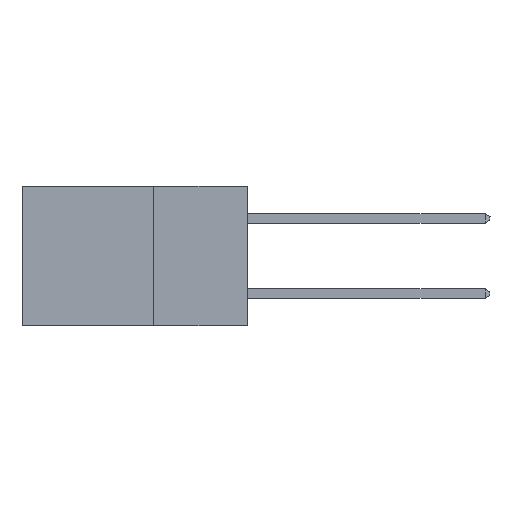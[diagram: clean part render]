
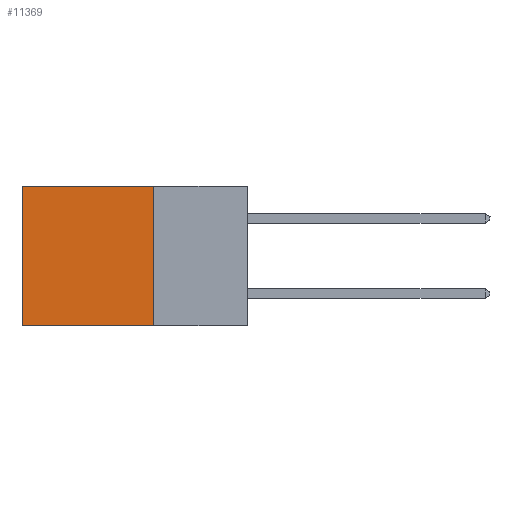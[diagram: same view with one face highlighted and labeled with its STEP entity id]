
A CAD part, left-side view. The second image highlights one B-rep face of the part: STEP entity #11369.
In plain terms, the highlighted planar face has unit normal (-1, 0, 0).
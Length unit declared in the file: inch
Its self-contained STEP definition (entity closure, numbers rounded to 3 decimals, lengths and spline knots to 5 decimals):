
#192 = DIRECTION ( 'NONE',  ( 0., 0., -1. ) ) ;
#212 = LINE ( 'NONE', #22846, #5450 ) ;
#910 = EDGE_CURVE ( 'NONE', #17585, #12472, #212, .T. ) ;
#913 = ORIENTED_EDGE ( 'NONE', *, *, #7001, .T. ) ;
#1144 = ORIENTED_EDGE ( 'NONE', *, *, #1780, .F. ) ;
#1780 = EDGE_CURVE ( 'NONE', #12472, #2490, #7830, .T. ) ;
#1997 = VECTOR ( 'NONE', #15049, 39.37008 ) ;
#2490 = VERTEX_POINT ( 'NONE', #12220 ) ;
#2828 = VERTEX_POINT ( 'NONE', #4873 ) ;
#3667 = CARTESIAN_POINT ( 'NONE',  ( 0.298, 0.6, 0. ) ) ;
#3754 = ORIENTED_EDGE ( 'NONE', *, *, #910, .F. ) ;
#4873 = CARTESIAN_POINT ( 'NONE',  ( 0.298, 0.6, 0. ) ) ;
#5029 = CARTESIAN_POINT ( 'NONE',  ( 0.298, 0.25, -0.37 ) ) ;
#5450 = VECTOR ( 'NONE', #24773, 39.37008 ) ;
#7001 = EDGE_CURVE ( 'NONE', #17585, #2828, #18368, .T. ) ;
#7830 = LINE ( 'NONE', #5029, #1997 ) ;
#8013 = PLANE ( 'NONE',  #23532 ) ;
#9423 = CARTESIAN_POINT ( 'NONE',  ( 0.298, 0.25, 0. ) ) ;
#9988 = CARTESIAN_POINT ( 'NONE',  ( 0.298, 0.25, 0. ) ) ;
#10891 = VECTOR ( 'NONE', #19261, 39.37008 ) ;
#11369 = ADVANCED_FACE ( 'NONE', ( #24390 ), #8013, .F. ) ;
#11377 = ORIENTED_EDGE ( 'NONE', *, *, #18677, .T. ) ;
#11971 = DIRECTION ( 'NONE',  ( 1., 0., 0. ) ) ;
#12220 = CARTESIAN_POINT ( 'NONE',  ( 0.298, 0.6, -0.37 ) ) ;
#12472 = VERTEX_POINT ( 'NONE', #17855 ) ;
#15049 = DIRECTION ( 'NONE',  ( 0., 1., 0. ) ) ;
#17585 = VERTEX_POINT ( 'NONE', #9423 ) ;
#17629 = DIRECTION ( 'NONE',  ( 0., 0., -1. ) ) ;
#17855 = CARTESIAN_POINT ( 'NONE',  ( 0.298, 0.25, -0.37 ) ) ;
#18368 = LINE ( 'NONE', #23260, #10891 ) ;
#18677 = EDGE_CURVE ( 'NONE', #2828, #2490, #24103, .T. ) ;
#19261 = DIRECTION ( 'NONE',  ( 0., 1., 0. ) ) ;
#22219 = VECTOR ( 'NONE', #17629, 39.37008 ) ;
#22846 = CARTESIAN_POINT ( 'NONE',  ( 0.298, 0.25, 0. ) ) ;
#23260 = CARTESIAN_POINT ( 'NONE',  ( 0.298, 0.25, 0. ) ) ;
#23532 = AXIS2_PLACEMENT_3D ( 'NONE', #9988, #11971, #192 ) ;
#23965 = EDGE_LOOP ( 'NONE', ( #11377, #1144, #3754, #913 ) ) ;
#24103 = LINE ( 'NONE', #3667, #22219 ) ;
#24390 = FACE_OUTER_BOUND ( 'NONE', #23965, .T. ) ;
#24773 = DIRECTION ( 'NONE',  ( 0., 0., -1. ) ) ;
